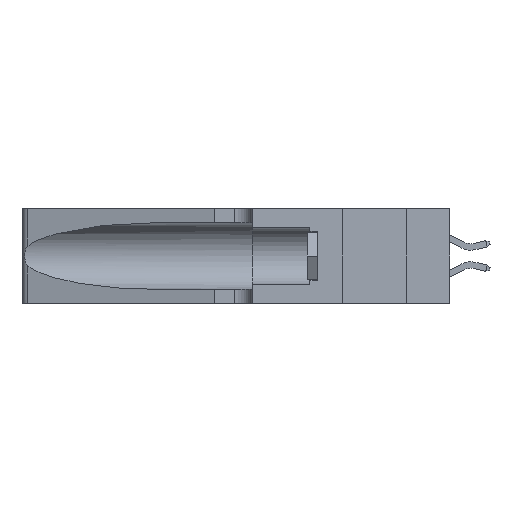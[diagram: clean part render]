
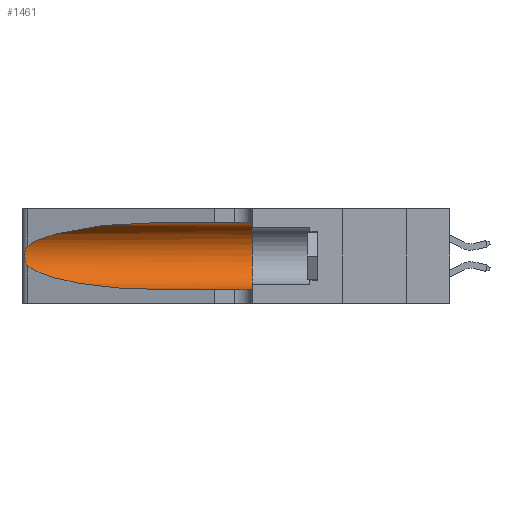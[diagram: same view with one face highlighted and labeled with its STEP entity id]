
A CAD part, left-side view. The second image highlights one B-rep face of the part: STEP entity #1461.
In plain terms, the highlighted cylindrical face has radius 3.308 mm (diameter 6.617 mm), a partial arc.
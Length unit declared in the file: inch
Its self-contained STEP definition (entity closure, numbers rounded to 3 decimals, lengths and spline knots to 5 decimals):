
#414 = VERTEX_POINT ( 'NONE', #21006 ) ;
#1109 = CARTESIAN_POINT ( 'NONE',  ( 0.26018, 1.23835, 0.19895 ) ) ;
#1254 = LINE ( 'NONE', #16212, #14178 ) ;
#1461 = ADVANCED_FACE ( 'NONE', ( #4215 ), #21506, .F. ) ;
#1861 = CARTESIAN_POINT ( 'NONE',  ( 0.25487, 1.22718, 0.22369 ) ) ;
#2507 = CARTESIAN_POINT ( 'NONE',  ( 0.1305, 0.72297, 0.31525 ) ) ;
#2795 = CARTESIAN_POINT ( 'NONE',  ( 0.1305, 0.35, 0.31525 ) ) ;
#2846 = CARTESIAN_POINT ( 'NONE',  ( 0.1305, 1.61858, 0.05475 ) ) ;
#2888 = LINE ( 'NONE', #2846, #11692 ) ;
#2933 = CARTESIAN_POINT ( 'NONE',  ( 0.26075, 1.23896, 0.178 ) ) ;
#3044 =( BOUNDED_CURVE ( )  B_SPLINE_CURVE ( 3, ( #20005, #7954, #21693, #11505 ),
 .UNSPECIFIED., .F., .F. ) 
 B_SPLINE_CURVE_WITH_KNOTS ( ( 4, 4 ),
 ( 3.44316, 4.71239 ),
 .UNSPECIFIED. ) 
 CURVE ( )  GEOMETRIC_REPRESENTATION_ITEM ( )  RATIONAL_B_SPLINE_CURVE ( ( 1., 0.87, 0.87, 1. ) ) 
 REPRESENTATION_ITEM ( '' )  );
#3731 =( BOUNDED_CURVE ( )  B_SPLINE_CURVE ( 3, ( #2507, #13034, #6042, #18160 ),
 .UNSPECIFIED., .F., .F. ) 
 B_SPLINE_CURVE_WITH_KNOTS ( ( 4, 4 ),
 ( 1.5708, 2.84003 ),
 .UNSPECIFIED. ) 
 CURVE ( )  GEOMETRIC_REPRESENTATION_ITEM ( )  RATIONAL_B_SPLINE_CURVE ( ( 1., 0.87, 0.87, 1. ) ) 
 REPRESENTATION_ITEM ( '' )  );
#3758 = EDGE_CURVE ( 'NONE', #414, #15317, #2888, .T. ) ;
#4215 = FACE_OUTER_BOUND ( 'NONE', #8087, .T. ) ;
#4679 = CARTESIAN_POINT ( 'NONE',  ( 0.25856, 1.23593, 0.16098 ) ) ;
#5000 = B_SPLINE_CURVE_WITH_KNOTS ( 'NONE', 3,
 ( #9943, #13354, #18499, #21875, #11701, #1109, #13421, #2933, #15172, #4679, #16883, #6448, #18574, #8229 ),
 .UNSPECIFIED., .F., .F.,
 ( 4, 2, 2, 2, 2, 2, 4 ),
 ( 0., 0.00027, 0.00053, 0.00107, 0.0016, 0.00187, 0.00214 ),
 .UNSPECIFIED. ) ;
#5549 = ORIENTED_EDGE ( 'NONE', *, *, #11656, .T. ) ;
#5711 = AXIS2_PLACEMENT_3D ( 'NONE', #9811, #21750, #11568 ) ;
#6004 = ORIENTED_EDGE ( 'NONE', *, *, #19237, .F. ) ;
#6042 = CARTESIAN_POINT ( 'NONE',  ( 0.2373, 1.15595, 0.28018 ) ) ;
#6354 = DIRECTION ( 'NONE',  ( 0., -1., 0. ) ) ;
#6448 = CARTESIAN_POINT ( 'NONE',  ( 0.25639, 1.23186, 0.15144 ) ) ;
#7032 = AXIS2_PLACEMENT_3D ( 'NONE', #7434, #10813, #11794 ) ;
#7434 = CARTESIAN_POINT ( 'NONE',  ( 0.1305, 1.61858, 0.185 ) ) ;
#7542 = DIRECTION ( 'NONE',  ( 0., -1., 0. ) ) ;
#7597 = ORIENTED_EDGE ( 'NONE', *, *, #8308, .T. ) ;
#7954 = CARTESIAN_POINT ( 'NONE',  ( 0.2373, 1.15595, 0.08982 ) ) ;
#8087 = EDGE_LOOP ( 'NONE', ( #5549, #7597, #11538, #13618, #6004, #13032 ) ) ;
#8229 = CARTESIAN_POINT ( 'NONE',  ( 0.25487, 1.22718, 0.14631 ) ) ;
#8308 = EDGE_CURVE ( 'NONE', #12117, #16216, #5000, .T. ) ;
#8400 = CARTESIAN_POINT ( 'NONE',  ( 0.1305, 0.35, 0.05475 ) ) ;
#9811 = CARTESIAN_POINT ( 'NONE',  ( 0.1305, 0.35, 0.185 ) ) ;
#9943 = CARTESIAN_POINT ( 'NONE',  ( 0.25487, 1.22718, 0.22369 ) ) ;
#10813 = DIRECTION ( 'NONE',  ( 0., -1., 0. ) ) ;
#11505 = CARTESIAN_POINT ( 'NONE',  ( 0.1305, 0.72297, 0.05475 ) ) ;
#11538 = ORIENTED_EDGE ( 'NONE', *, *, #17710, .T. ) ;
#11568 = DIRECTION ( 'NONE',  ( 0., 0., 1. ) ) ;
#11656 = EDGE_CURVE ( 'NONE', #22301, #12117, #3731, .T. ) ;
#11692 = VECTOR ( 'NONE', #6354, 39.37008 ) ;
#11701 = CARTESIAN_POINT ( 'NONE',  ( 0.25854, 1.2359, 0.20912 ) ) ;
#11794 = DIRECTION ( 'NONE',  ( 0., 0., -1. ) ) ;
#12117 = VERTEX_POINT ( 'NONE', #1861 ) ;
#13032 = ORIENTED_EDGE ( 'NONE', *, *, #13645, .F. ) ;
#13034 = CARTESIAN_POINT ( 'NONE',  ( 0.18966, 0.96281, 0.31525 ) ) ;
#13354 = CARTESIAN_POINT ( 'NONE',  ( 0.25555, 1.22994, 0.2215 ) ) ;
#13421 = CARTESIAN_POINT ( 'NONE',  ( 0.26075, 1.23896, 0.19203 ) ) ;
#13618 = ORIENTED_EDGE ( 'NONE', *, *, #3758, .T. ) ;
#13645 = EDGE_CURVE ( 'NONE', #22301, #21306, #1254, .T. ) ;
#14178 = VECTOR ( 'NONE', #7542, 39.37008 ) ;
#15172 = CARTESIAN_POINT ( 'NONE',  ( 0.26017, 1.23833, 0.17102 ) ) ;
#15317 = VERTEX_POINT ( 'NONE', #8400 ) ;
#16147 = CARTESIAN_POINT ( 'NONE',  ( 0.25487, 1.22718, 0.14631 ) ) ;
#16212 = CARTESIAN_POINT ( 'NONE',  ( 0.1305, 1.61858, 0.31525 ) ) ;
#16216 = VERTEX_POINT ( 'NONE', #16147 ) ;
#16883 = CARTESIAN_POINT ( 'NONE',  ( 0.25789, 1.23486, 0.15765 ) ) ;
#17012 = CIRCLE ( 'NONE', #5711, 0.13025 ) ;
#17170 = CARTESIAN_POINT ( 'NONE',  ( 0.1305, 0.72297, 0.31525 ) ) ;
#17710 = EDGE_CURVE ( 'NONE', #16216, #414, #3044, .T. ) ;
#18160 = CARTESIAN_POINT ( 'NONE',  ( 0.25487, 1.22718, 0.22369 ) ) ;
#18499 = CARTESIAN_POINT ( 'NONE',  ( 0.25639, 1.23184, 0.21858 ) ) ;
#18574 = CARTESIAN_POINT ( 'NONE',  ( 0.25555, 1.22993, 0.14849 ) ) ;
#19237 = EDGE_CURVE ( 'NONE', #21306, #15317, #17012, .T. ) ;
#20005 = CARTESIAN_POINT ( 'NONE',  ( 0.25487, 1.22718, 0.14631 ) ) ;
#21006 = CARTESIAN_POINT ( 'NONE',  ( 0.1305, 0.72297, 0.05475 ) ) ;
#21306 = VERTEX_POINT ( 'NONE', #2795 ) ;
#21506 = CYLINDRICAL_SURFACE ( 'NONE', #7032, 0.13025 ) ;
#21693 = CARTESIAN_POINT ( 'NONE',  ( 0.18966, 0.96281, 0.05475 ) ) ;
#21750 = DIRECTION ( 'NONE',  ( 0., 1., 0. ) ) ;
#21875 = CARTESIAN_POINT ( 'NONE',  ( 0.25787, 1.23484, 0.2124 ) ) ;
#22301 = VERTEX_POINT ( 'NONE', #17170 ) ;
